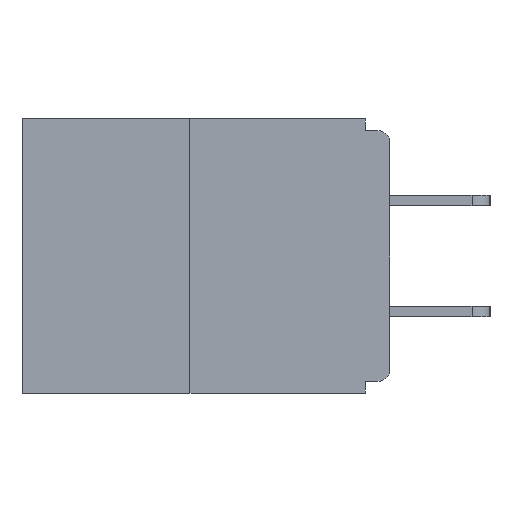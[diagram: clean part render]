
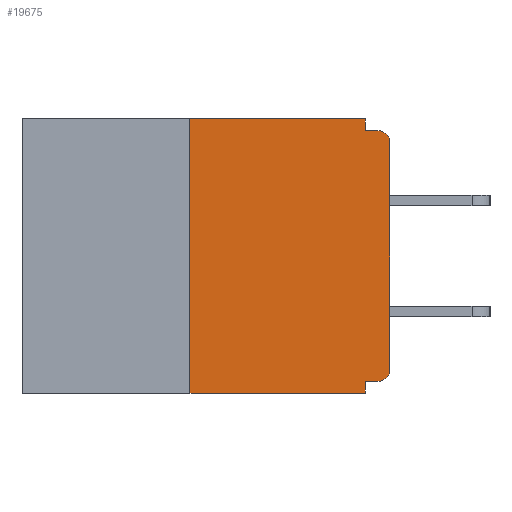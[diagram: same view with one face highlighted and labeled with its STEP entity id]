
A CAD part, left-side view. The second image highlights one B-rep face of the part: STEP entity #19675.
In plain terms, the highlighted planar face has unit normal (-1, 0, 0).
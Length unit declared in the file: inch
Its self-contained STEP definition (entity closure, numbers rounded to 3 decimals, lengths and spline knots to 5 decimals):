
#445 = DIRECTION ( 'NONE',  ( -1., 0., 0. ) ) ;
#981 = ORIENTED_EDGE ( 'NONE', *, *, #29542, .T. ) ;
#1687 = VECTOR ( 'NONE', #25122, 39.37008 ) ;
#1835 = LINE ( 'NONE', #20984, #27402 ) ;
#1875 = LINE ( 'NONE', #7704, #21251 ) ;
#2032 = AXIS2_PLACEMENT_3D ( 'NONE', #5052, #445, #7797 ) ;
#2234 = VERTEX_POINT ( 'NONE', #14571 ) ;
#3407 = VERTEX_POINT ( 'NONE', #19786 ) ;
#3851 = ORIENTED_EDGE ( 'NONE', *, *, #6246, .F. ) ;
#4635 = VERTEX_POINT ( 'NONE', #12084 ) ;
#5052 = CARTESIAN_POINT ( 'NONE',  ( 0., 0.015, -0.313 ) ) ;
#5273 = DIRECTION ( 'NONE',  ( 0., 0., -1. ) ) ;
#5555 = EDGE_CURVE ( 'NONE', #31656, #10534, #14332, .T. ) ;
#5910 = CARTESIAN_POINT ( 'NONE',  ( 0., 0.031, -0.343 ) ) ;
#6246 = EDGE_CURVE ( 'NONE', #4635, #15648, #26711, .T. ) ;
#6572 = ORIENTED_EDGE ( 'NONE', *, *, #15813, .T. ) ;
#7017 = EDGE_LOOP ( 'NONE', ( #16601, #8793, #7609, #3851, #30141, #981, #6572, #14526, #30991, #25549 ) ) ;
#7099 = DIRECTION ( 'NONE',  ( 0., -1., 0. ) ) ;
#7160 = AXIS2_PLACEMENT_3D ( 'NONE', #30017, #29807, #7567 ) ;
#7483 = EDGE_CURVE ( 'NONE', #31656, #15648, #16698, .T. ) ;
#7549 = VERTEX_POINT ( 'NONE', #8777 ) ;
#7567 = DIRECTION ( 'NONE',  ( 0., 0., -1. ) ) ;
#7609 = ORIENTED_EDGE ( 'NONE', *, *, #7483, .T. ) ;
#7635 = CARTESIAN_POINT ( 'NONE',  ( 0., 0.25, 0. ) ) ;
#7704 = CARTESIAN_POINT ( 'NONE',  ( 0., 0.031, 0. ) ) ;
#7797 = DIRECTION ( 'NONE',  ( 0., 0., -1. ) ) ;
#8123 = EDGE_CURVE ( 'NONE', #29414, #4635, #25997, .T. ) ;
#8777 = CARTESIAN_POINT ( 'NONE',  ( 0., 0.031, -0.015 ) ) ;
#8793 = ORIENTED_EDGE ( 'NONE', *, *, #5555, .F. ) ;
#8970 = VECTOR ( 'NONE', #19071, 39.37008 ) ;
#9340 = EDGE_CURVE ( 'NONE', #2234, #7549, #1875, .T. ) ;
#10034 = CARTESIAN_POINT ( 'NONE',  ( 0., 0.25, 0. ) ) ;
#10534 = VERTEX_POINT ( 'NONE', #10034 ) ;
#12084 = CARTESIAN_POINT ( 'NONE',  ( 0., 0.031, -0.328 ) ) ;
#12297 = DIRECTION ( 'NONE',  ( 0., 0., 1. ) ) ;
#12876 = CARTESIAN_POINT ( 'NONE',  ( 0., 0.46, 0. ) ) ;
#13595 = FACE_OUTER_BOUND ( 'NONE', #7017, .T. ) ;
#13659 = CARTESIAN_POINT ( 'NONE',  ( 0., 0.46, -0.343 ) ) ;
#13968 = CARTESIAN_POINT ( 'NONE',  ( 0., 0.015, -0.328 ) ) ;
#14188 = CIRCLE ( 'NONE', #2032, 0.015 ) ;
#14332 = LINE ( 'NONE', #7635, #18629 ) ;
#14526 = ORIENTED_EDGE ( 'NONE', *, *, #26620, .T. ) ;
#14571 = CARTESIAN_POINT ( 'NONE',  ( 0., 0.031, 0. ) ) ;
#14897 = PLANE ( 'NONE',  #7160 ) ;
#15417 = DIRECTION ( 'NONE',  ( 0., 1., 0. ) ) ;
#15648 = VERTEX_POINT ( 'NONE', #5910 ) ;
#15813 = EDGE_CURVE ( 'NONE', #3407, #22732, #1835, .T. ) ;
#16553 = DIRECTION ( 'NONE',  ( 0., 0., -1. ) ) ;
#16601 = ORIENTED_EDGE ( 'NONE', *, *, #17743, .F. ) ;
#16698 = LINE ( 'NONE', #13659, #8970 ) ;
#16946 = DIRECTION ( 'NONE',  ( 0., 0., -1. ) ) ;
#17111 = CIRCLE ( 'NONE', #25857, 0.015 ) ;
#17743 = EDGE_CURVE ( 'NONE', #10534, #2234, #29242, .T. ) ;
#18629 = VECTOR ( 'NONE', #12297, 39.37008 ) ;
#19071 = DIRECTION ( 'NONE',  ( 0., -1., 0. ) ) ;
#19349 = VECTOR ( 'NONE', #16553, 39.37008 ) ;
#19588 = CARTESIAN_POINT ( 'NONE',  ( 0., 0., -0.015 ) ) ;
#19675 = ADVANCED_FACE ( 'NONE', ( #13595 ), #14897, .F. ) ;
#19786 = CARTESIAN_POINT ( 'NONE',  ( 0., 0., -0.313 ) ) ;
#20733 = CARTESIAN_POINT ( 'NONE',  ( 0., 0.25, -0.343 ) ) ;
#20984 = CARTESIAN_POINT ( 'NONE',  ( 0., 0., 0. ) ) ;
#21251 = VECTOR ( 'NONE', #5273, 39.37008 ) ;
#21626 = VECTOR ( 'NONE', #7099, 39.37008 ) ;
#21821 = DIRECTION ( 'NONE',  ( -1., 0., 0. ) ) ;
#22009 = LINE ( 'NONE', #19588, #21626 ) ;
#22579 = CARTESIAN_POINT ( 'NONE',  ( 0., 0.015, -0.015 ) ) ;
#22732 = VERTEX_POINT ( 'NONE', #28205 ) ;
#24446 = VERTEX_POINT ( 'NONE', #22579 ) ;
#25122 = DIRECTION ( 'NONE',  ( 0., -1., 0. ) ) ;
#25141 = EDGE_CURVE ( 'NONE', #7549, #24446, #22009, .T. ) ;
#25549 = ORIENTED_EDGE ( 'NONE', *, *, #9340, .F. ) ;
#25631 = DIRECTION ( 'NONE',  ( 0., 0., 1. ) ) ;
#25857 = AXIS2_PLACEMENT_3D ( 'NONE', #31571, #21821, #16946 ) ;
#25997 = LINE ( 'NONE', #29978, #31033 ) ;
#26620 = EDGE_CURVE ( 'NONE', #22732, #24446, #17111, .T. ) ;
#26711 = LINE ( 'NONE', #27186, #19349 ) ;
#27186 = CARTESIAN_POINT ( 'NONE',  ( 0., 0.031, -0.343 ) ) ;
#27402 = VECTOR ( 'NONE', #25631, 39.37008 ) ;
#28205 = CARTESIAN_POINT ( 'NONE',  ( 0., 0., -0.03 ) ) ;
#29242 = LINE ( 'NONE', #12876, #1687 ) ;
#29414 = VERTEX_POINT ( 'NONE', #13968 ) ;
#29542 = EDGE_CURVE ( 'NONE', #29414, #3407, #14188, .T. ) ;
#29807 = DIRECTION ( 'NONE',  ( 1., 0., 0. ) ) ;
#29978 = CARTESIAN_POINT ( 'NONE',  ( 0., 0., -0.328 ) ) ;
#30017 = CARTESIAN_POINT ( 'NONE',  ( 0., 0.46, 0. ) ) ;
#30141 = ORIENTED_EDGE ( 'NONE', *, *, #8123, .F. ) ;
#30991 = ORIENTED_EDGE ( 'NONE', *, *, #25141, .F. ) ;
#31033 = VECTOR ( 'NONE', #15417, 39.37008 ) ;
#31571 = CARTESIAN_POINT ( 'NONE',  ( 0., 0.015, -0.03 ) ) ;
#31656 = VERTEX_POINT ( 'NONE', #20733 ) ;
